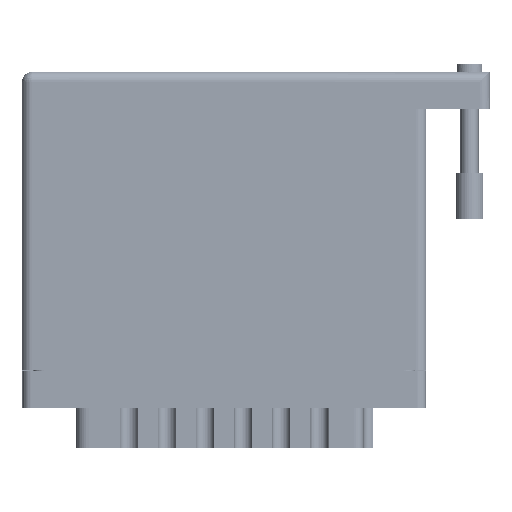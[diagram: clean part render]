
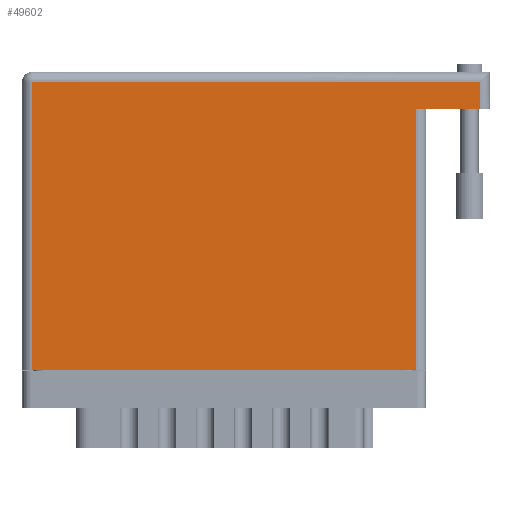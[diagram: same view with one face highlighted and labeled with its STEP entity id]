
A CAD part, front view. The second image highlights one B-rep face of the part: STEP entity #49602.
In plain terms, the highlighted face is planar.
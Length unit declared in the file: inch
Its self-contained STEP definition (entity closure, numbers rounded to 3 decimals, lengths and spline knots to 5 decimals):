
#172 = LINE ( 'NONE', #85699, #4871 ) ;
#970 = LINE ( 'NONE', #69070, #25502 ) ;
#1066 = AXIS2_PLACEMENT_3D ( 'NONE', #33649, #12792, #71353 ) ;
#4050 = DIRECTION ( 'NONE',  ( -1., 0., 0. ) ) ;
#4871 = VECTOR ( 'NONE', #4050, 39.37008 ) ;
#6927 = CARTESIAN_POINT ( 'NONE',  ( 2.685, 1.774, 0. ) ) ;
#10157 = DIRECTION ( 'NONE',  ( 0., 1., 0. ) ) ;
#12792 = DIRECTION ( 'NONE',  ( 0., 0., -1. ) ) ;
#14543 = LINE ( 'NONE', #15014, #36678 ) ;
#15014 = CARTESIAN_POINT ( 'NONE',  ( 3.12, 2.03, 0. ) ) ;
#17966 = CARTESIAN_POINT ( 'NONE',  ( 2.685, 1.774, 0. ) ) ;
#18330 = DIRECTION ( 'NONE',  ( 1., 0., 0. ) ) ;
#19309 = PLANE ( 'NONE',  #1066 ) ;
#20510 = CARTESIAN_POINT ( 'NONE',  ( 0.07, 0., 0. ) ) ;
#21293 = VERTEX_POINT ( 'NONE', #30442 ) ;
#22346 = VERTEX_POINT ( 'NONE', #87818 ) ;
#22558 = FACE_OUTER_BOUND ( 'NONE', #68613, .T. ) ;
#24258 = ORIENTED_EDGE ( 'NONE', *, *, #30926, .T. ) ;
#25322 = VERTEX_POINT ( 'NONE', #6927 ) ;
#25502 = VECTOR ( 'NONE', #18330, 39.37008 ) ;
#29205 = EDGE_CURVE ( 'NONE', #21293, #52921, #970, .T. ) ;
#29902 = ORIENTED_EDGE ( 'NONE', *, *, #29205, .T. ) ;
#30442 = CARTESIAN_POINT ( 'NONE',  ( 0.07, 0., 0. ) ) ;
#30926 = EDGE_CURVE ( 'NONE', #90384, #22346, #14543, .T. ) ;
#33649 = CARTESIAN_POINT ( 'NONE',  ( 0., 2.03, 0. ) ) ;
#36678 = VECTOR ( 'NONE', #60591, 39.37008 ) ;
#37456 = CARTESIAN_POINT ( 'NONE',  ( 0.07, 1.96, 0. ) ) ;
#38908 = LINE ( 'NONE', #17966, #56396 ) ;
#42940 = DIRECTION ( 'NONE',  ( 0., -1., 0. ) ) ;
#48555 = VECTOR ( 'NONE', #42940, 39.37008 ) ;
#48798 = LINE ( 'NONE', #92499, #91776 ) ;
#49602 = ADVANCED_FACE ( 'NONE', ( #22558 ), #19309, .F. ) ;
#49704 = LINE ( 'NONE', #20510, #48555 ) ;
#52921 = VERTEX_POINT ( 'NONE', #81206 ) ;
#55791 = DIRECTION ( 'NONE',  ( -1., 0., 0. ) ) ;
#56396 = VECTOR ( 'NONE', #10157, 39.37008 ) ;
#60591 = DIRECTION ( 'NONE',  ( 0., 1., 0. ) ) ;
#62011 = ORIENTED_EDGE ( 'NONE', *, *, #80599, .T. ) ;
#68613 = EDGE_LOOP ( 'NONE', ( #29902, #73118, #80454, #24258, #62011, #77528 ) ) ;
#69070 = CARTESIAN_POINT ( 'NONE',  ( 0., 0., 0. ) ) ;
#71353 = DIRECTION ( 'NONE',  ( -1., 0., 0. ) ) ;
#71848 = EDGE_CURVE ( 'NONE', #52921, #25322, #38908, .T. ) ;
#73118 = ORIENTED_EDGE ( 'NONE', *, *, #71848, .T. ) ;
#75992 = EDGE_CURVE ( 'NONE', #95448, #21293, #49704, .T. ) ;
#77528 = ORIENTED_EDGE ( 'NONE', *, *, #75992, .T. ) ;
#80454 = ORIENTED_EDGE ( 'NONE', *, *, #90786, .F. ) ;
#80599 = EDGE_CURVE ( 'NONE', #22346, #95448, #48798, .T. ) ;
#81206 = CARTESIAN_POINT ( 'NONE',  ( 2.685, 0., 0. ) ) ;
#85699 = CARTESIAN_POINT ( 'NONE',  ( 3.19, 1.774, 0. ) ) ;
#87818 = CARTESIAN_POINT ( 'NONE',  ( 3.12, 1.96, 0. ) ) ;
#90384 = VERTEX_POINT ( 'NONE', #90405 ) ;
#90405 = CARTESIAN_POINT ( 'NONE',  ( 3.12, 1.774, 0. ) ) ;
#90786 = EDGE_CURVE ( 'NONE', #90384, #25322, #172, .T. ) ;
#91776 = VECTOR ( 'NONE', #55791, 39.37008 ) ;
#92499 = CARTESIAN_POINT ( 'NONE',  ( 0., 1.96, 0. ) ) ;
#95448 = VERTEX_POINT ( 'NONE', #37456 ) ;
